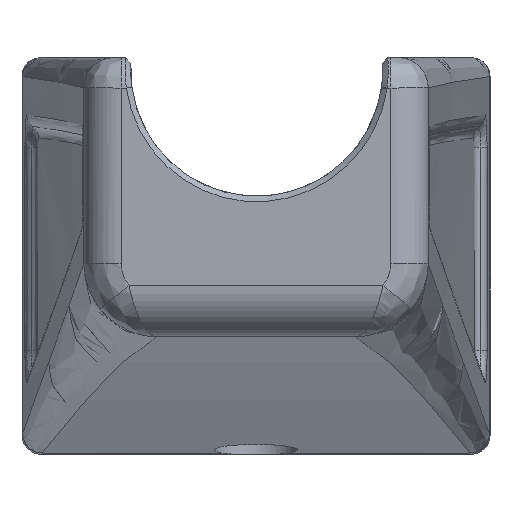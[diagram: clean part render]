
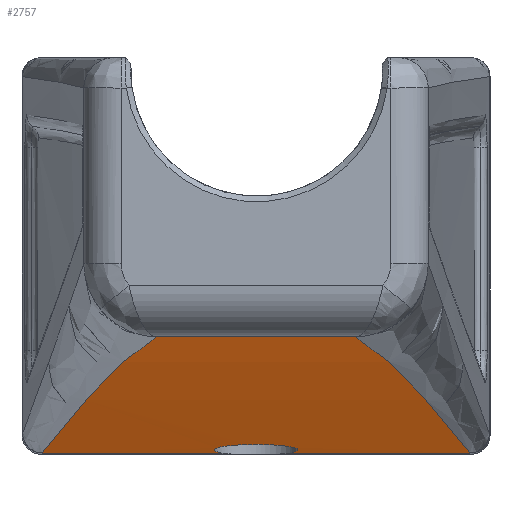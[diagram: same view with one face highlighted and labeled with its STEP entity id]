
A CAD part, front view. The second image highlights one B-rep face of the part: STEP entity #2757.
In plain terms, the highlighted cylindrical face has radius 1594.73 mm (diameter 3189.46 mm), a partial arc.
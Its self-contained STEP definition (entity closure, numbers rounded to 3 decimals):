
#108=B_SPLINE_CURVE_WITH_KNOTS('',3,(#3541,#3542,#3543,#3544,#3545,#3546,
#3547,#3548,#3549,#3550,#3551,#3552,#3553,#3554,#3555,#3556,#3557,#3558,
#3559,#3560,#3561,#3562,#3563),.UNSPECIFIED.,.F.,.F.,(4,2,2,2,2,2,3,2,2,
2,4),(-0.946,-0.852,-0.681,-0.51,
-0.339,-0.169,0.,0.17,0.34,
0.51,0.681),.UNSPECIFIED.);
#110=B_SPLINE_CURVE_WITH_KNOTS('',3,(#3579,#3580,#3581,#3582,#3583,#3584),
 .UNSPECIFIED.,.F.,.F.,(4,2,4),(0.681,0.851,0.946),
 .UNSPECIFIED.);
#237=B_SPLINE_CURVE_WITH_KNOTS('',3,(#6411,#6412,#6413,#6414),
 .UNSPECIFIED.,.F.,.F.,(4,4),(-0.316,-0.304),
 .UNSPECIFIED.);
#240=B_SPLINE_CURVE_WITH_KNOTS('',3,(#6899,#6900,#6901,#6902),
 .UNSPECIFIED.,.F.,.F.,(4,4),(-15.111,-0.316),
 .UNSPECIFIED.);
#250=B_SPLINE_CURVE_WITH_KNOTS('',3,(#7198,#7199,#7200,#7201),
 .UNSPECIFIED.,.F.,.F.,(4,4),(-0.316,-0.304),
 .UNSPECIFIED.);
#255=B_SPLINE_CURVE_WITH_KNOTS('',3,(#7676,#7677,#7678,#7679),
 .UNSPECIFIED.,.F.,.F.,(4,4),(-15.111,-0.316),
 .UNSPECIFIED.);
#262=LINE('',#3591,#412);
#264=LINE('',#3742,#414);
#409=LINE('',#7871,#559);
#412=VECTOR('',#2993,10.);
#414=VECTOR('',#2995,10.);
#559=VECTOR('',#3528,10.);
#599=CYLINDRICAL_SURFACE('',#2973,1594.729);
#777=FACE_OUTER_BOUND('',#955,.T.);
#955=EDGE_LOOP('',(#2531,#2532,#2533,#2534,#2535,#2536,#2537,#2538,#2539));
#1062=VERTEX_POINT('',#3538);
#1063=VERTEX_POINT('',#3540);
#1064=VERTEX_POINT('',#3564);
#1066=VERTEX_POINT('',#3590);
#1071=VERTEX_POINT('',#3695);
#1301=VERTEX_POINT('',#6397);
#1303=VERTEX_POINT('',#6898);
#1305=VERTEX_POINT('',#7190);
#1307=VERTEX_POINT('',#7667);
#1311=EDGE_CURVE('',#1063,#1062,#108,.T.);
#1313=EDGE_CURVE('',#1062,#1064,#110,.T.);
#1316=EDGE_CURVE('',#1066,#1063,#262,.T.);
#1322=EDGE_CURVE('',#1064,#1071,#264,.T.);
#1689=EDGE_CURVE('',#1301,#1066,#237,.T.);
#1692=EDGE_CURVE('',#1303,#1301,#240,.T.);
#1707=EDGE_CURVE('',#1305,#1071,#250,.T.);
#1712=EDGE_CURVE('',#1307,#1305,#255,.T.);
#1719=EDGE_CURVE('',#1307,#1303,#409,.T.);
#2531=ORIENTED_EDGE('',*,*,#1311,.T.);
#2532=ORIENTED_EDGE('',*,*,#1313,.T.);
#2533=ORIENTED_EDGE('',*,*,#1322,.T.);
#2534=ORIENTED_EDGE('',*,*,#1707,.F.);
#2535=ORIENTED_EDGE('',*,*,#1712,.F.);
#2536=ORIENTED_EDGE('',*,*,#1719,.T.);
#2537=ORIENTED_EDGE('',*,*,#1692,.T.);
#2538=ORIENTED_EDGE('',*,*,#1689,.T.);
#2539=ORIENTED_EDGE('',*,*,#1316,.T.);
#2757=ADVANCED_FACE('',(#777),#599,.F.);
#2973=AXIS2_PLACEMENT_3D('',#7870,#3526,#3527);
#2993=DIRECTION('',(1.,0.,0.));
#2995=DIRECTION('',(1.,0.,0.));
#3526=DIRECTION('center_axis',(-1.,0.,0.));
#3527=DIRECTION('ref_axis',(0.,0.131,0.991));
#3528=DIRECTION('',(-1.,0.,0.));
#3538=CARTESIAN_POINT('',(20.477,-31.891,-156.922));
#3540=CARTESIAN_POINT('',(12.295,-29.303,-157.26));
#3541=CARTESIAN_POINT('Ctrl Pts',(12.295,-29.303,-157.26));
#3542=CARTESIAN_POINT('Ctrl Pts',(12.108,-29.57,-157.225));
#3543=CARTESIAN_POINT('Ctrl Pts',(11.947,-29.861,-157.187));
#3544=CARTESIAN_POINT('Ctrl Pts',(11.59,-30.722,-157.074));
#3545=CARTESIAN_POINT('Ctrl Pts',(11.477,-31.325,-156.995));
#3546=CARTESIAN_POINT('Ctrl Pts',(11.477,-32.456,-156.848));
#3547=CARTESIAN_POINT('Ctrl Pts',(11.59,-33.059,-156.77));
#3548=CARTESIAN_POINT('Ctrl Pts',(12.05,-34.17,-156.627));
#3549=CARTESIAN_POINT('Ctrl Pts',(12.398,-34.677,-156.562));
#3550=CARTESIAN_POINT('Ctrl Pts',(13.198,-35.475,-156.46));
#3551=CARTESIAN_POINT('Ctrl Pts',(13.703,-35.82,-156.416));
#3552=CARTESIAN_POINT('Ctrl Pts',(14.81,-36.278,-156.357));
#3553=CARTESIAN_POINT('Ctrl Pts',(15.412,-36.391,-156.343));
#3554=CARTESIAN_POINT('Ctrl Pts',(15.977,-36.391,-156.343));
#3555=CARTESIAN_POINT('Ctrl Pts',(16.543,-36.391,-156.343));
#3556=CARTESIAN_POINT('Ctrl Pts',(17.146,-36.277,-156.357));
#3557=CARTESIAN_POINT('Ctrl Pts',(18.255,-35.817,-156.416));
#3558=CARTESIAN_POINT('Ctrl Pts',(18.76,-35.471,-156.46));
#3559=CARTESIAN_POINT('Ctrl Pts',(19.559,-34.672,-156.562));
#3560=CARTESIAN_POINT('Ctrl Pts',(19.905,-34.165,-156.627));
#3561=CARTESIAN_POINT('Ctrl Pts',(20.364,-33.057,-156.77));
#3562=CARTESIAN_POINT('Ctrl Pts',(20.477,-32.454,-156.848));
#3563=CARTESIAN_POINT('Ctrl Pts',(20.477,-31.891,-156.922));
#3564=CARTESIAN_POINT('',(19.658,-29.303,-157.26));
#3579=CARTESIAN_POINT('Ctrl Pts',(20.477,-31.891,-156.922));
#3580=CARTESIAN_POINT('Ctrl Pts',(20.477,-31.326,-156.995));
#3581=CARTESIAN_POINT('Ctrl Pts',(20.364,-30.724,-157.074));
#3582=CARTESIAN_POINT('Ctrl Pts',(20.008,-29.863,-157.186));
#3583=CARTESIAN_POINT('Ctrl Pts',(19.846,-29.571,-157.225));
#3584=CARTESIAN_POINT('Ctrl Pts',(19.658,-29.303,-157.26));
#3590=CARTESIAN_POINT('',(-6.934,-29.303,-157.26));
#3591=CARTESIAN_POINT('',(-9.1,-29.303,-157.26));
#3695=CARTESIAN_POINT('',(38.888,-29.303,-157.26));
#3742=CARTESIAN_POINT('',(-9.1,-29.303,-157.26));
#6397=CARTESIAN_POINT('',(-6.923,-29.418,-157.245));
#6411=CARTESIAN_POINT('Ctrl Pts',(-6.923,-29.418,-157.245));
#6412=CARTESIAN_POINT('Ctrl Pts',(-6.927,-29.38,-157.25));
#6413=CARTESIAN_POINT('Ctrl Pts',(-6.931,-29.342,-157.255));
#6414=CARTESIAN_POINT('Ctrl Pts',(-6.934,-29.303,-157.26));
#6898=CARTESIAN_POINT('',(5.283,-175.713,-144.808));
#6899=CARTESIAN_POINT('Ctrl Pts',(5.283,-175.713,-144.808));
#6900=CARTESIAN_POINT('Ctrl Pts',(2.12,-126.802,-146.705));
#6901=CARTESIAN_POINT('Ctrl Pts',(-1.963,-77.965,-150.856));
#6902=CARTESIAN_POINT('Ctrl Pts',(-6.923,-29.418,-157.245));
#7190=CARTESIAN_POINT('',(38.876,-29.418,-157.245));
#7198=CARTESIAN_POINT('Ctrl Pts',(38.876,-29.418,-157.245));
#7199=CARTESIAN_POINT('Ctrl Pts',(38.88,-29.38,-157.25));
#7200=CARTESIAN_POINT('Ctrl Pts',(38.884,-29.342,-157.255));
#7201=CARTESIAN_POINT('Ctrl Pts',(38.888,-29.303,-157.26));
#7667=CARTESIAN_POINT('',(26.67,-175.713,-144.808));
#7676=CARTESIAN_POINT('Ctrl Pts',(26.67,-175.713,-144.808));
#7677=CARTESIAN_POINT('Ctrl Pts',(29.834,-126.802,-146.705));
#7678=CARTESIAN_POINT('Ctrl Pts',(33.916,-77.965,-150.856));
#7679=CARTESIAN_POINT('Ctrl Pts',(38.876,-29.418,-157.245));
#7870=CARTESIAN_POINT('Origin',(41.053,-237.506,-1738.339));
#7871=CARTESIAN_POINT('',(-9.1,-175.713,-144.808));
